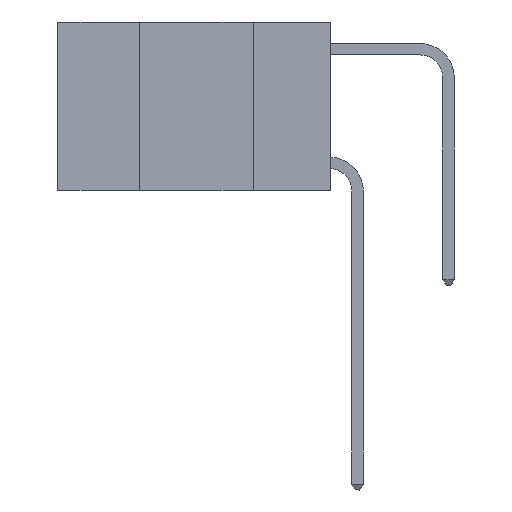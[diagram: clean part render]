
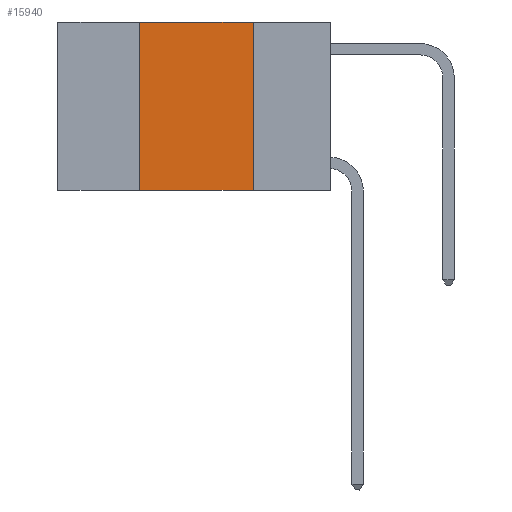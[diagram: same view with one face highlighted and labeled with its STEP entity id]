
A CAD part, left-side view. The second image highlights one B-rep face of the part: STEP entity #15940.
In plain terms, the highlighted planar face has unit normal (-1, 0, 0).
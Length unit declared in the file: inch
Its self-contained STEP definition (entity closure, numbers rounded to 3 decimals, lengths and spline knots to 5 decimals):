
#167 = CARTESIAN_POINT ( 'NONE',  ( 0., 0.6, 0. ) ) ;
#360 = CARTESIAN_POINT ( 'NONE',  ( 0., 0.42, 0. ) ) ;
#472 = EDGE_CURVE ( 'NONE', #7173, #14202, #3826, .T. ) ;
#1504 = VECTOR ( 'NONE', #14940, 39.37008 ) ;
#1519 = PLANE ( 'NONE',  #9961 ) ;
#2380 = LINE ( 'NONE', #16371, #1504 ) ;
#3040 = DIRECTION ( 'NONE',  ( 0., 0., -1. ) ) ;
#3571 = ORIENTED_EDGE ( 'NONE', *, *, #17492, .F. ) ;
#3685 = VERTEX_POINT ( 'NONE', #19168 ) ;
#3826 = LINE ( 'NONE', #167, #10945 ) ;
#3858 = DIRECTION ( 'NONE',  ( 0., 0., 1. ) ) ;
#5674 = ORIENTED_EDGE ( 'NONE', *, *, #12415, .T. ) ;
#6303 = ORIENTED_EDGE ( 'NONE', *, *, #16315, .F. ) ;
#6692 = CARTESIAN_POINT ( 'NONE',  ( 0., 0.17, 0. ) ) ;
#7173 = VERTEX_POINT ( 'NONE', #360 ) ;
#7223 = VECTOR ( 'NONE', #7928, 39.37008 ) ;
#7714 = VECTOR ( 'NONE', #3858, 39.37008 ) ;
#7928 = DIRECTION ( 'NONE',  ( 0., 0., -1. ) ) ;
#9052 = CARTESIAN_POINT ( 'NONE',  ( 0., 0.6, 0. ) ) ;
#9895 = CARTESIAN_POINT ( 'NONE',  ( 0., 0.42, 0. ) ) ;
#9961 = AXIS2_PLACEMENT_3D ( 'NONE', #9052, #12103, #3040 ) ;
#10687 = CARTESIAN_POINT ( 'NONE',  ( 0., 0.42, -0.37 ) ) ;
#10945 = VECTOR ( 'NONE', #11872, 39.37008 ) ;
#11265 = LINE ( 'NONE', #16840, #7223 ) ;
#11745 = LINE ( 'NONE', #9895, #7714 ) ;
#11872 = DIRECTION ( 'NONE',  ( 0., -1., 0. ) ) ;
#12103 = DIRECTION ( 'NONE',  ( 1., 0., 0. ) ) ;
#12415 = EDGE_CURVE ( 'NONE', #16641, #3685, #2380, .T. ) ;
#14202 = VERTEX_POINT ( 'NONE', #6692 ) ;
#14444 = ORIENTED_EDGE ( 'NONE', *, *, #472, .F. ) ;
#14771 = FACE_OUTER_BOUND ( 'NONE', #15977, .T. ) ;
#14940 = DIRECTION ( 'NONE',  ( 0., -1., 0. ) ) ;
#15940 = ADVANCED_FACE ( 'NONE', ( #14771 ), #1519, .F. ) ;
#15977 = EDGE_LOOP ( 'NONE', ( #3571, #14444, #6303, #5674 ) ) ;
#16315 = EDGE_CURVE ( 'NONE', #16641, #7173, #11745, .T. ) ;
#16371 = CARTESIAN_POINT ( 'NONE',  ( 0., 0.6, -0.37 ) ) ;
#16641 = VERTEX_POINT ( 'NONE', #10687 ) ;
#16840 = CARTESIAN_POINT ( 'NONE',  ( 0., 0.17, 0. ) ) ;
#17492 = EDGE_CURVE ( 'NONE', #14202, #3685, #11265, .T. ) ;
#19168 = CARTESIAN_POINT ( 'NONE',  ( 0., 0.17, -0.37 ) ) ;
